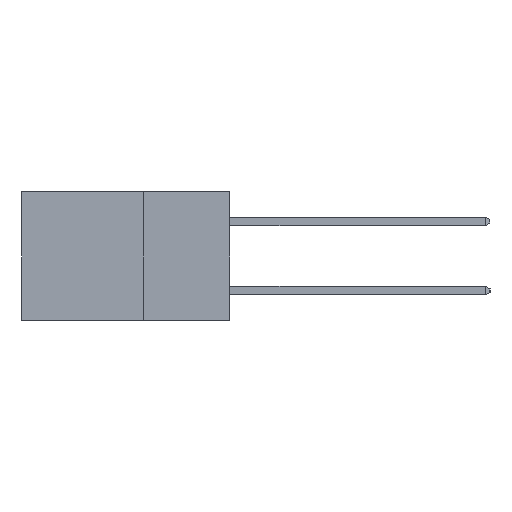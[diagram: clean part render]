
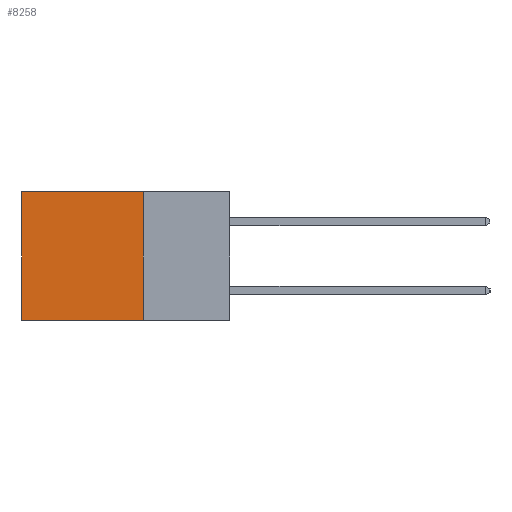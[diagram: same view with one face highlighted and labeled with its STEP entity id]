
A CAD part, left-side view. The second image highlights one B-rep face of the part: STEP entity #8258.
In plain terms, the highlighted planar face has unit normal (-1, 0, 0).
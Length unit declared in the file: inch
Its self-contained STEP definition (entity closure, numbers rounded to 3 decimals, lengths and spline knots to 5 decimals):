
#1127 = CARTESIAN_POINT ( 'NONE',  ( 0.2615, 0.25, 0. ) ) ;
#1190 = VECTOR ( 'NONE', #11015, 39.37008 ) ;
#2558 = ORIENTED_EDGE ( 'NONE', *, *, #21674, .T. ) ;
#2804 = CARTESIAN_POINT ( 'NONE',  ( 0.2615, 0.25, -0.37 ) ) ;
#3501 = CARTESIAN_POINT ( 'NONE',  ( 0.2615, 0.25, -0.37 ) ) ;
#3786 = VECTOR ( 'NONE', #17138, 39.37008 ) ;
#4729 = EDGE_LOOP ( 'NONE', ( #12042, #13209, #4763, #2558 ) ) ;
#4763 = ORIENTED_EDGE ( 'NONE', *, *, #6772, .F. ) ;
#5583 = LINE ( 'NONE', #3501, #20559 ) ;
#5678 = DIRECTION ( 'NONE',  ( 0., 0., -1. ) ) ;
#6772 = EDGE_CURVE ( 'NONE', #8373, #21091, #5583, .T. ) ;
#6800 = DIRECTION ( 'NONE',  ( 0., 0., -1. ) ) ;
#6926 = AXIS2_PLACEMENT_3D ( 'NONE', #2804, #18483, #6800 ) ;
#7070 = CARTESIAN_POINT ( 'NONE',  ( 0.2615, 0.25, 0. ) ) ;
#8141 = VECTOR ( 'NONE', #5678, 39.37008 ) ;
#8258 = ADVANCED_FACE ( 'NONE', ( #18049 ), #10662, .F. ) ;
#8373 = VERTEX_POINT ( 'NONE', #1127 ) ;
#9650 = LINE ( 'NONE', #21119, #3786 ) ;
#10662 = PLANE ( 'NONE',  #6926 ) ;
#11015 = DIRECTION ( 'NONE',  ( 0., 1., 0. ) ) ;
#12042 = ORIENTED_EDGE ( 'NONE', *, *, #15664, .T. ) ;
#12732 = LINE ( 'NONE', #15439, #8141 ) ;
#13209 = ORIENTED_EDGE ( 'NONE', *, *, #16301, .F. ) ;
#13340 = CARTESIAN_POINT ( 'NONE',  ( 0.2615, 0.25, -0.37 ) ) ;
#15439 = CARTESIAN_POINT ( 'NONE',  ( 0.2615, 0.6, -0.37 ) ) ;
#15664 = EDGE_CURVE ( 'NONE', #21193, #16814, #12732, .T. ) ;
#16301 = EDGE_CURVE ( 'NONE', #21091, #16814, #9650, .T. ) ;
#16814 = VERTEX_POINT ( 'NONE', #20331 ) ;
#16898 = LINE ( 'NONE', #7070, #1190 ) ;
#17138 = DIRECTION ( 'NONE',  ( 0., 1., 0. ) ) ;
#18049 = FACE_OUTER_BOUND ( 'NONE', #4729, .T. ) ;
#18483 = DIRECTION ( 'NONE',  ( 1., 0., 0. ) ) ;
#19138 = DIRECTION ( 'NONE',  ( 0., 0., -1. ) ) ;
#20331 = CARTESIAN_POINT ( 'NONE',  ( 0.2615, 0.6, -0.37 ) ) ;
#20559 = VECTOR ( 'NONE', #19138, 39.37008 ) ;
#21091 = VERTEX_POINT ( 'NONE', #13340 ) ;
#21119 = CARTESIAN_POINT ( 'NONE',  ( 0.2615, 0.25, -0.37 ) ) ;
#21193 = VERTEX_POINT ( 'NONE', #21412 ) ;
#21412 = CARTESIAN_POINT ( 'NONE',  ( 0.2615, 0.6, 0. ) ) ;
#21674 = EDGE_CURVE ( 'NONE', #8373, #21193, #16898, .T. ) ;
